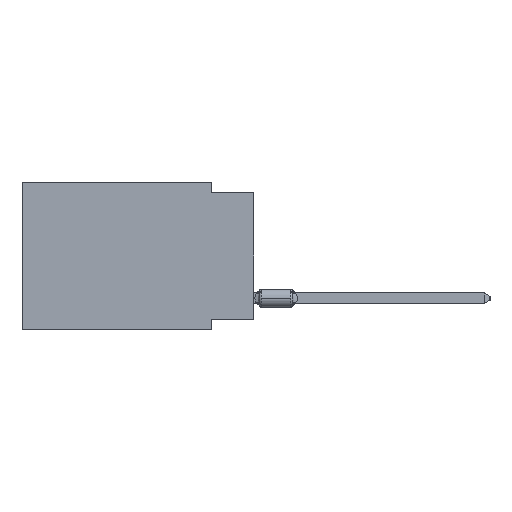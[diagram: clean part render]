
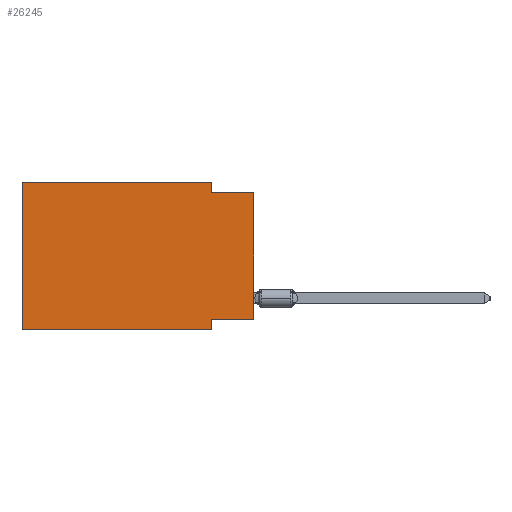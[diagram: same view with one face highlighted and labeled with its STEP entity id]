
A CAD part, left-side view. The second image highlights one B-rep face of the part: STEP entity #26245.
In plain terms, the highlighted planar face has unit normal (-1, 0, 0).
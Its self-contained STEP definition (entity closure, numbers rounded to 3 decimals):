
#12 = VECTOR ( 'NONE', #18602, 1000. ) ;
#1110 = DIRECTION ( 'NONE',  ( 1., 0., 0. ) ) ;
#1676 = EDGE_CURVE ( 'NONE', #33452, #20932, #7334, .T. ) ;
#1767 = LINE ( 'NONE', #24357, #22688 ) ;
#2117 = LINE ( 'NONE', #36217, #31402 ) ;
#3206 = EDGE_CURVE ( 'NONE', #6296, #20932, #29082, .T. ) ;
#4601 = CARTESIAN_POINT ( 'NONE',  ( 0., 2.54, -0.635 ) ) ;
#4874 = EDGE_CURVE ( 'NONE', #33452, #32748, #2117, .T. ) ;
#5217 = CARTESIAN_POINT ( 'NONE',  ( 0., 2.54, 0. ) ) ;
#5885 = CARTESIAN_POINT ( 'NONE',  ( 0., 13.97, 0. ) ) ;
#5976 = LINE ( 'NONE', #25226, #10031 ) ;
#6181 = VECTOR ( 'NONE', #8689, 1000. ) ;
#6296 = VERTEX_POINT ( 'NONE', #23735 ) ;
#7215 = PLANE ( 'NONE',  #8538 ) ;
#7334 = LINE ( 'NONE', #32727, #12 ) ;
#8538 = AXIS2_PLACEMENT_3D ( 'NONE', #21091, #1110, #24230 ) ;
#8689 = DIRECTION ( 'NONE',  ( 0., 0., -1. ) ) ;
#9453 = DIRECTION ( 'NONE',  ( 0., 0., -1. ) ) ;
#10031 = VECTOR ( 'NONE', #31002, 1000. ) ;
#11097 = ORIENTED_EDGE ( 'NONE', *, *, #4874, .F. ) ;
#11673 = CARTESIAN_POINT ( 'NONE',  ( 0., 2.54, -8.89 ) ) ;
#12311 = EDGE_CURVE ( 'NONE', #31639, #34078, #12484, .T. ) ;
#12484 = LINE ( 'NONE', #23769, #14222 ) ;
#12509 = CARTESIAN_POINT ( 'NONE',  ( 0., 2.54, -8.89 ) ) ;
#13734 = VECTOR ( 'NONE', #9453, 1000. ) ;
#14222 = VECTOR ( 'NONE', #35114, 1000. ) ;
#15359 = EDGE_CURVE ( 'NONE', #20282, #31639, #19961, .T. ) ;
#16027 = EDGE_LOOP ( 'NONE', ( #16225, #35126, #20678, #19742, #11097, #30449, #33521, #35221 ) ) ;
#16225 = ORIENTED_EDGE ( 'NONE', *, *, #20999, .T. ) ;
#18602 = DIRECTION ( 'NONE',  ( 0., -1., 0. ) ) ;
#18815 = CARTESIAN_POINT ( 'NONE',  ( 0., 0., -0.635 ) ) ;
#19673 = DIRECTION ( 'NONE',  ( 0., 0., 1. ) ) ;
#19742 = ORIENTED_EDGE ( 'NONE', *, *, #31891, .F. ) ;
#19961 = LINE ( 'NONE', #34094, #6181 ) ;
#20282 = VERTEX_POINT ( 'NONE', #5217 ) ;
#20678 = ORIENTED_EDGE ( 'NONE', *, *, #15359, .F. ) ;
#20932 = VERTEX_POINT ( 'NONE', #12509 ) ;
#20999 = EDGE_CURVE ( 'NONE', #26598, #34078, #1767, .T. ) ;
#21091 = CARTESIAN_POINT ( 'NONE',  ( 0., 13.97, 0. ) ) ;
#22688 = VECTOR ( 'NONE', #35704, 1000. ) ;
#22808 = LINE ( 'NONE', #30813, #30765 ) ;
#23735 = CARTESIAN_POINT ( 'NONE',  ( 0., 2.54, -8.255 ) ) ;
#23769 = CARTESIAN_POINT ( 'NONE',  ( 0., 0., -0.635 ) ) ;
#24230 = DIRECTION ( 'NONE',  ( 0., 0., -1. ) ) ;
#24357 = CARTESIAN_POINT ( 'NONE',  ( 0., 0., 0. ) ) ;
#25226 = CARTESIAN_POINT ( 'NONE',  ( 0., 13.97, 0. ) ) ;
#26245 = ADVANCED_FACE ( 'NONE', ( #26285 ), #7215, .F. ) ;
#26285 = FACE_OUTER_BOUND ( 'NONE', #16027, .T. ) ;
#26598 = VERTEX_POINT ( 'NONE', #33067 ) ;
#27834 = DIRECTION ( 'NONE',  ( 0., 1., 0. ) ) ;
#29082 = LINE ( 'NONE', #11673, #13734 ) ;
#30449 = ORIENTED_EDGE ( 'NONE', *, *, #1676, .T. ) ;
#30765 = VECTOR ( 'NONE', #27834, 1000. ) ;
#30813 = CARTESIAN_POINT ( 'NONE',  ( 0., 0., -8.255 ) ) ;
#31002 = DIRECTION ( 'NONE',  ( 0., -1., 0. ) ) ;
#31402 = VECTOR ( 'NONE', #19673, 1000. ) ;
#31639 = VERTEX_POINT ( 'NONE', #4601 ) ;
#31891 = EDGE_CURVE ( 'NONE', #32748, #20282, #5976, .T. ) ;
#32727 = CARTESIAN_POINT ( 'NONE',  ( 0., 13.97, -8.89 ) ) ;
#32748 = VERTEX_POINT ( 'NONE', #5885 ) ;
#32902 = CARTESIAN_POINT ( 'NONE',  ( 0., 13.97, -8.89 ) ) ;
#33067 = CARTESIAN_POINT ( 'NONE',  ( 0., 0., -8.255 ) ) ;
#33452 = VERTEX_POINT ( 'NONE', #32902 ) ;
#33521 = ORIENTED_EDGE ( 'NONE', *, *, #3206, .F. ) ;
#34078 = VERTEX_POINT ( 'NONE', #18815 ) ;
#34094 = CARTESIAN_POINT ( 'NONE',  ( 0., 2.54, 0. ) ) ;
#35114 = DIRECTION ( 'NONE',  ( 0., -1., 0. ) ) ;
#35126 = ORIENTED_EDGE ( 'NONE', *, *, #12311, .F. ) ;
#35221 = ORIENTED_EDGE ( 'NONE', *, *, #35927, .F. ) ;
#35704 = DIRECTION ( 'NONE',  ( 0., 0., 1. ) ) ;
#35927 = EDGE_CURVE ( 'NONE', #26598, #6296, #22808, .T. ) ;
#36217 = CARTESIAN_POINT ( 'NONE',  ( 0., 13.97, 0. ) ) ;
